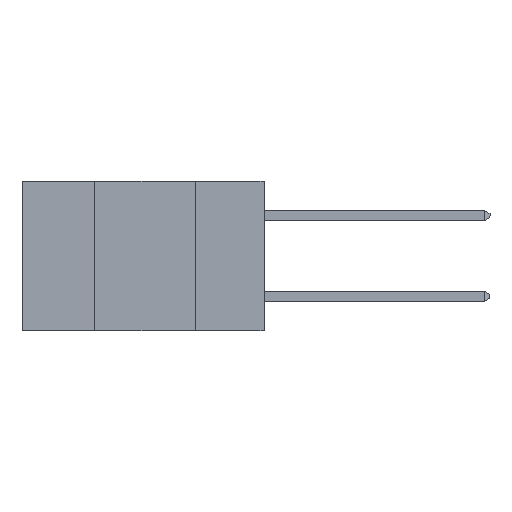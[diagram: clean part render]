
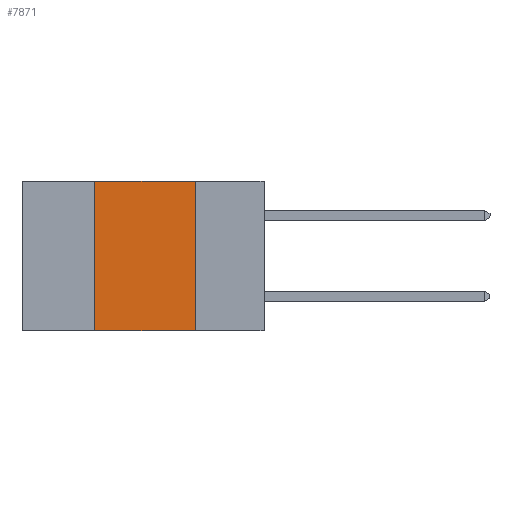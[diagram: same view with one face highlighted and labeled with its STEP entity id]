
A CAD part, left-side view. The second image highlights one B-rep face of the part: STEP entity #7871.
In plain terms, the highlighted planar face has unit normal (-1, 0, 0).
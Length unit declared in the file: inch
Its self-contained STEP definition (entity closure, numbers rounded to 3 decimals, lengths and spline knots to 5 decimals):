
#378 = EDGE_LOOP ( 'NONE', ( #8633, #8644, #9016, #9368 ) ) ;
#661 = CARTESIAN_POINT ( 'NONE',  ( 0., 0.17, -0.37 ) ) ;
#1222 = CARTESIAN_POINT ( 'NONE',  ( 0., 0.6, 0. ) ) ;
#1438 = DIRECTION ( 'NONE',  ( 0., -1., 0. ) ) ;
#1894 = VECTOR ( 'NONE', #1438, 39.37008 ) ;
#2138 = DIRECTION ( 'NONE',  ( 1., 0., 0. ) ) ;
#2446 = CARTESIAN_POINT ( 'NONE',  ( 0., 0.17, 0. ) ) ;
#2457 = EDGE_CURVE ( 'NONE', #7387, #8562, #11244, .T. ) ;
#2466 = VECTOR ( 'NONE', #4152, 39.37008 ) ;
#2711 = EDGE_CURVE ( 'NONE', #8562, #5011, #8922, .T. ) ;
#3113 = EDGE_CURVE ( 'NONE', #7387, #9411, #7160, .T. ) ;
#3449 = CARTESIAN_POINT ( 'NONE',  ( 0., 0.17, 0. ) ) ;
#3682 = AXIS2_PLACEMENT_3D ( 'NONE', #1222, #2138, #8300 ) ;
#3785 = CARTESIAN_POINT ( 'NONE',  ( 0., 0.6, -0.37 ) ) ;
#4152 = DIRECTION ( 'NONE',  ( 0., -1., 0. ) ) ;
#5011 = VERTEX_POINT ( 'NONE', #2446 ) ;
#5240 = CARTESIAN_POINT ( 'NONE',  ( 0., 0.6, 0. ) ) ;
#5704 = CARTESIAN_POINT ( 'NONE',  ( 0., 0.42, 0. ) ) ;
#5760 = CARTESIAN_POINT ( 'NONE',  ( 0., 0.42, 0. ) ) ;
#6286 = FACE_OUTER_BOUND ( 'NONE', #378, .T. ) ;
#7160 = LINE ( 'NONE', #3785, #2466 ) ;
#7387 = VERTEX_POINT ( 'NONE', #10020 ) ;
#7871 = ADVANCED_FACE ( 'NONE', ( #6286 ), #10785, .F. ) ;
#8300 = DIRECTION ( 'NONE',  ( 0., 0., -1. ) ) ;
#8444 = VECTOR ( 'NONE', #9556, 39.37008 ) ;
#8562 = VERTEX_POINT ( 'NONE', #5760 ) ;
#8633 = ORIENTED_EDGE ( 'NONE', *, *, #8781, .F. ) ;
#8644 = ORIENTED_EDGE ( 'NONE', *, *, #2711, .F. ) ;
#8781 = EDGE_CURVE ( 'NONE', #5011, #9411, #10410, .T. ) ;
#8922 = LINE ( 'NONE', #5240, #1894 ) ;
#9016 = ORIENTED_EDGE ( 'NONE', *, *, #2457, .F. ) ;
#9064 = VECTOR ( 'NONE', #10110, 39.37008 ) ;
#9368 = ORIENTED_EDGE ( 'NONE', *, *, #3113, .T. ) ;
#9411 = VERTEX_POINT ( 'NONE', #661 ) ;
#9556 = DIRECTION ( 'NONE',  ( 0., 0., -1. ) ) ;
#10020 = CARTESIAN_POINT ( 'NONE',  ( 0., 0.42, -0.37 ) ) ;
#10110 = DIRECTION ( 'NONE',  ( 0., 0., 1. ) ) ;
#10410 = LINE ( 'NONE', #3449, #8444 ) ;
#10785 = PLANE ( 'NONE',  #3682 ) ;
#11244 = LINE ( 'NONE', #5704, #9064 ) ;
